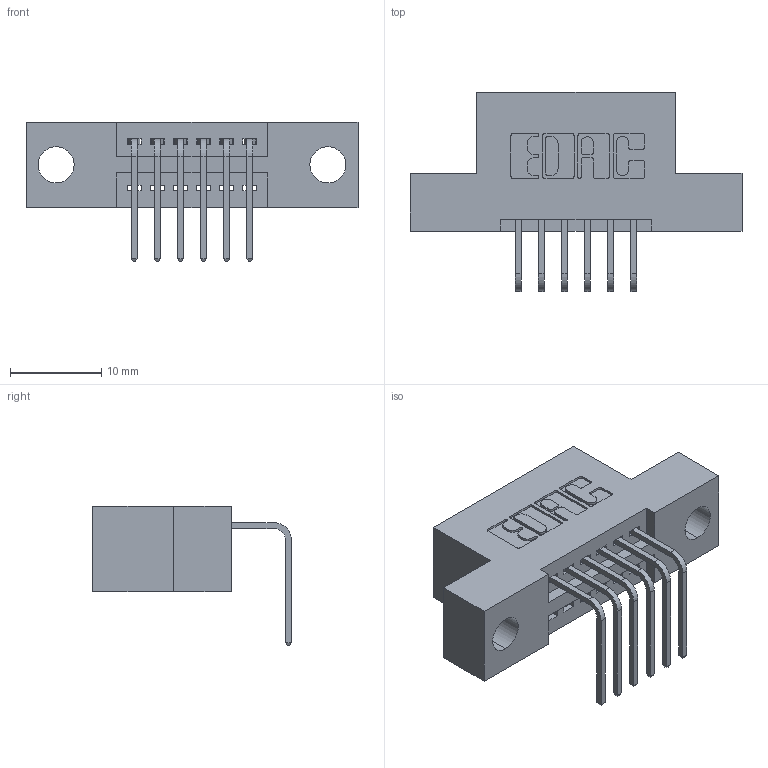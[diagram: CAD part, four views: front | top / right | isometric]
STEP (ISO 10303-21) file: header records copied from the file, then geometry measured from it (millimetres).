
FILE_DESCRIPTION (( 'STEP AP203' ), '1' );
FILE_NAME ('345-006-558-104.STEP', '2021-06-01T16:06:26', ( '' ), ( '' ), 'SwSTEP 2.0', 'SolidWorks 2020', '' );
FILE_SCHEMA (( 'CONFIG_CONTROL_DESIGN' ));
Length unit declared in the file: inch
Products named in the file (3): 345 Part_Flush Mounting Lugs - 0.156 Dia-TI; 345-292-001_558 Tail - 2; 345-006-558-104
Assembly tree (7 placements, depth 2):
  345-006-558-104
    345 Part_Flush Mounting Lugs - 0.156 Dia-TI
    345-292-001_558 Tail - 2  x6
Bounding box: 36.45 x 21.83 x 15.37 mm (x, y, z)
Volume: 3081.1 mm3; surface area: 3565.2 mm2
Topology: 7 solids, 7 shells, 500 faces, 1469 edges, 970 vertices
Faces by surface type: plane 346, cylinder 154
Entity records: 9865 total; most frequent: CARTESIAN_POINT 1720, ORIENTED_EDGE 1658, DIRECTION 1553, EDGE_CURVE 829, LINE 673, VECTOR 673, VERTEX_POINT 550, AXIS2_PLACEMENT_3D 440
